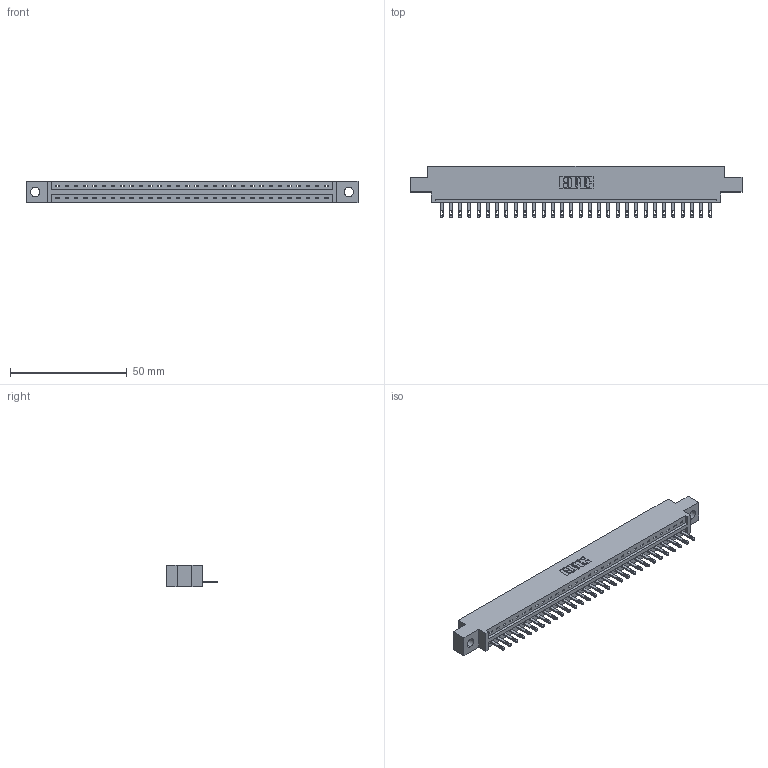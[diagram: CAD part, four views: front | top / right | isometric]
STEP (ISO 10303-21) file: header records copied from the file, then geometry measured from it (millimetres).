
FILE_DESCRIPTION (( 'STEP AP203' ), '1' );
FILE_NAME ('337-030-500-604.STEP', '2019-09-30T23:08:11', ( '' ), ( '' ), 'SwSTEP 2.0', 'SolidWorks 2016', '' );
FILE_SCHEMA (( 'CONFIG_CONTROL_DESIGN' ));
Length unit declared in the file: inch
Products named in the file (3): 337-030-500-604; 337 Part_0.170 Offset - 0.156 Dia-TH; 345-292-001_345-293-100
Assembly tree (31 placements, depth 2):
  337-030-500-604
    337 Part_0.170 Offset - 0.156 Dia-TH
    345-292-001_345-293-100  x30
Bounding box: 141.88 x 21.85 x 9.4 mm (x, y, z)
Volume: 14409.5 mm3; surface area: 14785.3 mm2
Topology: 31 solids, 31 shells, 1858 faces, 5723 edges, 3814 vertices
Faces by surface type: plane 1274, cylinder 584
Entity records: 23917 total; most frequent: CARTESIAN_POINT 4172, ORIENTED_EDGE 4138, DIRECTION 3537, EDGE_CURVE 2069, VECTOR 1937, LINE 1937, VERTEX_POINT 1378, AXIS2_PLACEMENT_3D 800
